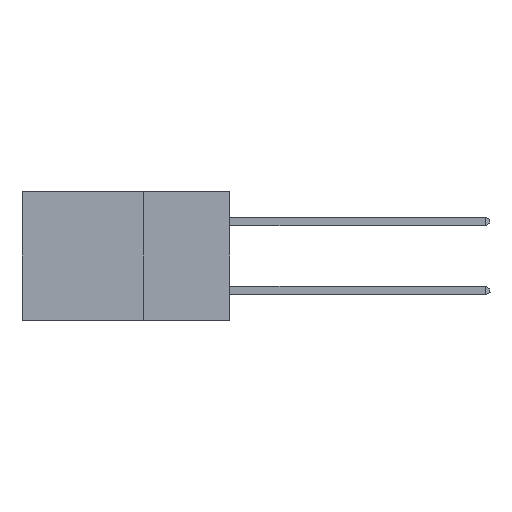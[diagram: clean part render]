
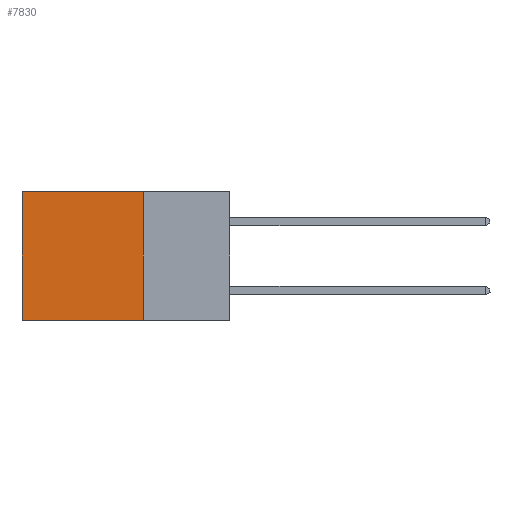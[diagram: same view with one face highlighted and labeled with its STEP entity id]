
A CAD part, left-side view. The second image highlights one B-rep face of the part: STEP entity #7830.
In plain terms, the highlighted planar face has unit normal (-1, 0, 0).
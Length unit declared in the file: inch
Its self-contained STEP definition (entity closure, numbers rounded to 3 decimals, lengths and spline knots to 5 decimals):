
#953 = PLANE ( 'NONE',  #4135 ) ;
#1264 = ORIENTED_EDGE ( 'NONE', *, *, #1269, .T. ) ;
#1269 = EDGE_CURVE ( 'NONE', #11279, #2453, #2826, .T. ) ;
#1469 = CARTESIAN_POINT ( 'NONE',  ( 0.298, 0.25, -0.37 ) ) ;
#1676 = VECTOR ( 'NONE', #6184, 39.37008 ) ;
#2009 = EDGE_CURVE ( 'NONE', #2453, #5529, #4319, .T. ) ;
#2185 = ORIENTED_EDGE ( 'NONE', *, *, #2009, .T. ) ;
#2453 = VERTEX_POINT ( 'NONE', #9380 ) ;
#2535 = FACE_OUTER_BOUND ( 'NONE', #3164, .T. ) ;
#2826 = LINE ( 'NONE', #10203, #10489 ) ;
#3058 = DIRECTION ( 'NONE',  ( 0., 0., -1. ) ) ;
#3164 = EDGE_LOOP ( 'NONE', ( #2185, #11417, #11228, #1264 ) ) ;
#3451 = VECTOR ( 'NONE', #8558, 39.37008 ) ;
#3663 = VERTEX_POINT ( 'NONE', #4591 ) ;
#3667 = LINE ( 'NONE', #5874, #8670 ) ;
#4135 = AXIS2_PLACEMENT_3D ( 'NONE', #7984, #7851, #9887 ) ;
#4319 = LINE ( 'NONE', #12220, #1676 ) ;
#4591 = CARTESIAN_POINT ( 'NONE',  ( 0.298, 0.25, -0.37 ) ) ;
#5529 = VERTEX_POINT ( 'NONE', #10672 ) ;
#5874 = CARTESIAN_POINT ( 'NONE',  ( 0.298, 0.25, 0. ) ) ;
#6184 = DIRECTION ( 'NONE',  ( 0., 0., -1. ) ) ;
#7064 = LINE ( 'NONE', #1469, #3451 ) ;
#7830 = ADVANCED_FACE ( 'NONE', ( #2535 ), #953, .F. ) ;
#7851 = DIRECTION ( 'NONE',  ( 1., 0., 0. ) ) ;
#7984 = CARTESIAN_POINT ( 'NONE',  ( 0.298, 0.25, 0. ) ) ;
#8130 = EDGE_CURVE ( 'NONE', #3663, #5529, #7064, .T. ) ;
#8558 = DIRECTION ( 'NONE',  ( 0., 1., 0. ) ) ;
#8670 = VECTOR ( 'NONE', #3058, 39.37008 ) ;
#9380 = CARTESIAN_POINT ( 'NONE',  ( 0.298, 0.6, 0. ) ) ;
#9410 = CARTESIAN_POINT ( 'NONE',  ( 0.298, 0.25, 0. ) ) ;
#9887 = DIRECTION ( 'NONE',  ( 0., 0., -1. ) ) ;
#10203 = CARTESIAN_POINT ( 'NONE',  ( 0.298, 0.25, 0. ) ) ;
#10246 = DIRECTION ( 'NONE',  ( 0., 1., 0. ) ) ;
#10489 = VECTOR ( 'NONE', #10246, 39.37008 ) ;
#10672 = CARTESIAN_POINT ( 'NONE',  ( 0.298, 0.6, -0.37 ) ) ;
#11228 = ORIENTED_EDGE ( 'NONE', *, *, #11925, .F. ) ;
#11279 = VERTEX_POINT ( 'NONE', #9410 ) ;
#11417 = ORIENTED_EDGE ( 'NONE', *, *, #8130, .F. ) ;
#11925 = EDGE_CURVE ( 'NONE', #11279, #3663, #3667, .T. ) ;
#12220 = CARTESIAN_POINT ( 'NONE',  ( 0.298, 0.6, 0. ) ) ;
